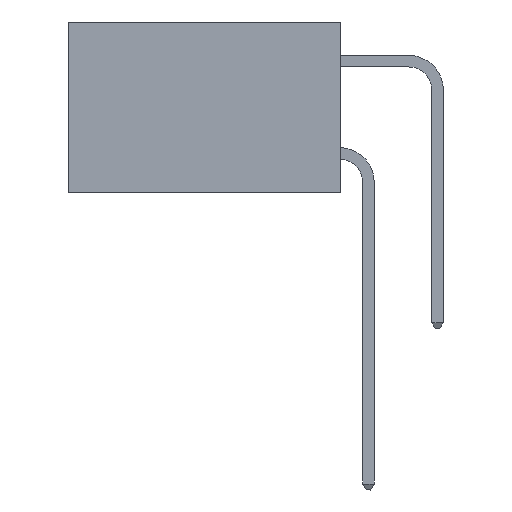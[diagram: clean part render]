
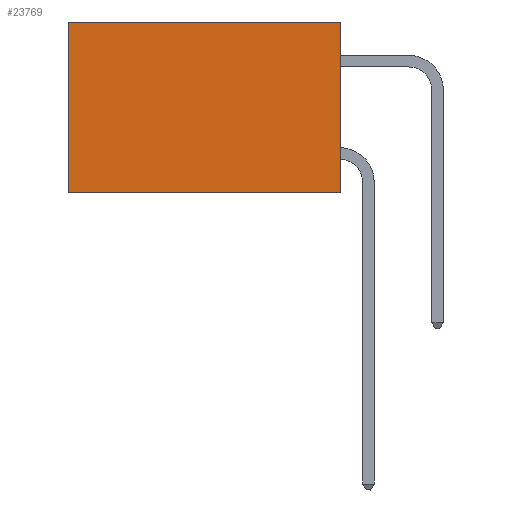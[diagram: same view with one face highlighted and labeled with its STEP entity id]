
A CAD part, left-side view. The second image highlights one B-rep face of the part: STEP entity #23769.
In plain terms, the highlighted planar face has unit normal (-1, 0, 0).
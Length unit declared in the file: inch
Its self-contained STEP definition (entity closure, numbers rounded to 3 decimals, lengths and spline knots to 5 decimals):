
#45 = VECTOR ( 'NONE', #7241, 39.37008 ) ;
#498 = EDGE_LOOP ( 'NONE', ( #16724, #25887, #35841, #24024 ) ) ;
#1530 = DIRECTION ( 'NONE',  ( 0., 0., -1. ) ) ;
#2422 = LINE ( 'NONE', #24505, #30426 ) ;
#4399 = CARTESIAN_POINT ( 'NONE',  ( 0.277, 0., -0.37 ) ) ;
#4715 = VECTOR ( 'NONE', #5166, 39.37008 ) ;
#4996 = CARTESIAN_POINT ( 'NONE',  ( 0.277, 0.59, 0. ) ) ;
#5166 = DIRECTION ( 'NONE',  ( 0., 1., 0. ) ) ;
#7084 = PLANE ( 'NONE',  #23879 ) ;
#7241 = DIRECTION ( 'NONE',  ( 0., 0., -1. ) ) ;
#9333 = EDGE_CURVE ( 'NONE', #30211, #22633, #2422, .T. ) ;
#12530 = EDGE_CURVE ( 'NONE', #26535, #32490, #22416, .T. ) ;
#12574 = FACE_OUTER_BOUND ( 'NONE', #498, .T. ) ;
#13624 = CARTESIAN_POINT ( 'NONE',  ( 0.277, 0., -0.37 ) ) ;
#13871 = LINE ( 'NONE', #18849, #19485 ) ;
#16044 = DIRECTION ( 'NONE',  ( 0., 0., -1. ) ) ;
#16724 = ORIENTED_EDGE ( 'NONE', *, *, #9333, .T. ) ;
#18309 = DIRECTION ( 'NONE',  ( 1., 0., 0. ) ) ;
#18849 = CARTESIAN_POINT ( 'NONE',  ( 0.277, 0., 0. ) ) ;
#19192 = CARTESIAN_POINT ( 'NONE',  ( 0.277, 0., 0. ) ) ;
#19485 = VECTOR ( 'NONE', #21708, 39.37008 ) ;
#21708 = DIRECTION ( 'NONE',  ( 0., 1., 0. ) ) ;
#21917 = EDGE_CURVE ( 'NONE', #32490, #22633, #33567, .T. ) ;
#22416 = LINE ( 'NONE', #4399, #45 ) ;
#22633 = VERTEX_POINT ( 'NONE', #30112 ) ;
#23769 = ADVANCED_FACE ( 'NONE', ( #12574 ), #7084, .F. ) ;
#23879 = AXIS2_PLACEMENT_3D ( 'NONE', #35000, #18309, #1530 ) ;
#24024 = ORIENTED_EDGE ( 'NONE', *, *, #28943, .T. ) ;
#24505 = CARTESIAN_POINT ( 'NONE',  ( 0.277, 0.59, -0.37 ) ) ;
#25887 = ORIENTED_EDGE ( 'NONE', *, *, #21917, .F. ) ;
#26535 = VERTEX_POINT ( 'NONE', #19192 ) ;
#28943 = EDGE_CURVE ( 'NONE', #26535, #30211, #13871, .T. ) ;
#30112 = CARTESIAN_POINT ( 'NONE',  ( 0.277, 0.59, -0.37 ) ) ;
#30211 = VERTEX_POINT ( 'NONE', #4996 ) ;
#30426 = VECTOR ( 'NONE', #16044, 39.37008 ) ;
#31106 = CARTESIAN_POINT ( 'NONE',  ( 0.277, 0., -0.37 ) ) ;
#32490 = VERTEX_POINT ( 'NONE', #31106 ) ;
#33567 = LINE ( 'NONE', #13624, #4715 ) ;
#35000 = CARTESIAN_POINT ( 'NONE',  ( 0.277, 0., -0.37 ) ) ;
#35841 = ORIENTED_EDGE ( 'NONE', *, *, #12530, .F. ) ;
